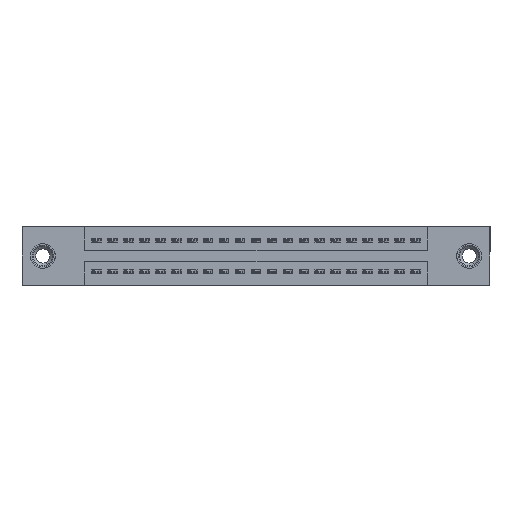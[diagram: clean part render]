
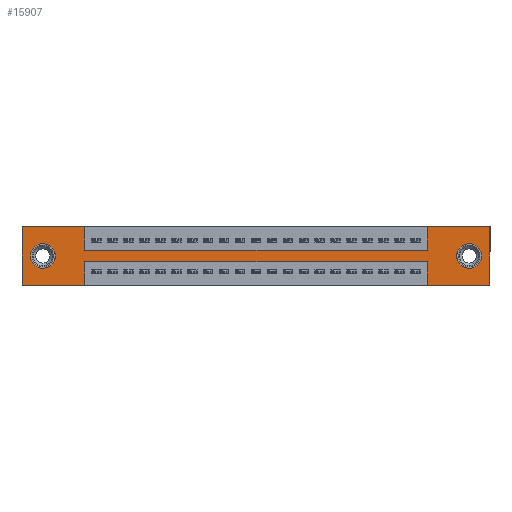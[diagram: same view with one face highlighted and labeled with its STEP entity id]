
A CAD part, front view. The second image highlights one B-rep face of the part: STEP entity #15907.
In plain terms, the highlighted planar face has unit normal (0, -1, 0).
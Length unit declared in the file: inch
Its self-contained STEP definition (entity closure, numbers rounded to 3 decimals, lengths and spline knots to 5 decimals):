
#292 = DIRECTION ( 'NONE',  ( 0., 0., -1. ) ) ;
#305 = CARTESIAN_POINT ( 'NONE',  ( 0., 0., -0.37 ) ) ;
#357 = CARTESIAN_POINT ( 'NONE',  ( 0., 0., 0. ) ) ;
#392 = CARTESIAN_POINT ( 'NONE',  ( 2.5425, 0., 0. ) ) ;
#472 = DIRECTION ( 'NONE',  ( 0., 0., -1. ) ) ;
#495 = CARTESIAN_POINT ( 'NONE',  ( 2.935, 0., 0. ) ) ;
#607 = DIRECTION ( 'NONE',  ( 1., 0., 0. ) ) ;
#788 = EDGE_CURVE ( 'NONE', #6210, #15255, #9337, .T. ) ;
#856 = CARTESIAN_POINT ( 'NONE',  ( 0.13, 0., -0.263 ) ) ;
#1022 = AXIS2_PLACEMENT_3D ( 'NONE', #18558, #13735, #15409 ) ;
#1032 = CIRCLE ( 'NONE', #16692, 0.078 ) ;
#1078 = VECTOR ( 'NONE', #10219, 39.37008 ) ;
#1104 = ORIENTED_EDGE ( 'NONE', *, *, #15872, .F. ) ;
#1366 = EDGE_CURVE ( 'NONE', #14508, #17656, #20268, .T. ) ;
#1466 = DIRECTION ( 'NONE',  ( 0., 0., 1. ) ) ;
#1497 = EDGE_CURVE ( 'NONE', #8282, #8139, #3645, .T. ) ;
#1965 = CARTESIAN_POINT ( 'NONE',  ( 0.3925, 0., -0.22 ) ) ;
#2150 = EDGE_CURVE ( 'NONE', #5523, #16238, #2598, .T. ) ;
#2354 = VERTEX_POINT ( 'NONE', #9370 ) ;
#2570 = ORIENTED_EDGE ( 'NONE', *, *, #788, .F. ) ;
#2598 = LINE ( 'NONE', #8615, #6475 ) ;
#2851 = EDGE_CURVE ( 'NONE', #16183, #10274, #19952, .T. ) ;
#3087 = CARTESIAN_POINT ( 'NONE',  ( 0.13, 0., -0.185 ) ) ;
#3565 = DIRECTION ( 'NONE',  ( 0., 0., -1. ) ) ;
#3645 = LINE ( 'NONE', #14074, #12171 ) ;
#3792 = VECTOR ( 'NONE', #1466, 39.37008 ) ;
#3975 = ORIENTED_EDGE ( 'NONE', *, *, #12436, .F. ) ;
#4322 = ORIENTED_EDGE ( 'NONE', *, *, #5326, .T. ) ;
#4615 = CARTESIAN_POINT ( 'NONE',  ( 0.3925, 0., -0.37 ) ) ;
#4636 = EDGE_CURVE ( 'NONE', #20492, #5523, #18578, .T. ) ;
#4645 = EDGE_LOOP ( 'NONE', ( #10405, #4322 ) ) ;
#4746 = VERTEX_POINT ( 'NONE', #856 ) ;
#4771 = CARTESIAN_POINT ( 'NONE',  ( 2.5425, 0., -0.37 ) ) ;
#4886 = CIRCLE ( 'NONE', #1022, 0.078 ) ;
#5216 = CARTESIAN_POINT ( 'NONE',  ( 2.5425, 0., -0.22 ) ) ;
#5326 = EDGE_CURVE ( 'NONE', #17656, #14508, #20364, .T. ) ;
#5474 = AXIS2_PLACEMENT_3D ( 'NONE', #8737, #10388, #292 ) ;
#5523 = VERTEX_POINT ( 'NONE', #4615 ) ;
#5547 = CARTESIAN_POINT ( 'NONE',  ( 2.5425, 0., 0. ) ) ;
#5802 = LINE ( 'NONE', #18113, #21106 ) ;
#6210 = VERTEX_POINT ( 'NONE', #5547 ) ;
#6363 = VERTEX_POINT ( 'NONE', #357 ) ;
#6380 = VECTOR ( 'NONE', #10973, 39.37008 ) ;
#6475 = VECTOR ( 'NONE', #10263, 39.37008 ) ;
#6629 = VECTOR ( 'NONE', #15482, 39.37008 ) ;
#6963 = VECTOR ( 'NONE', #11293, 39.37008 ) ;
#6988 = EDGE_LOOP ( 'NONE', ( #13357, #9820 ) ) ;
#7296 = ORIENTED_EDGE ( 'NONE', *, *, #12013, .F. ) ;
#7413 = LINE ( 'NONE', #19263, #6380 ) ;
#8139 = VERTEX_POINT ( 'NONE', #5216 ) ;
#8282 = VERTEX_POINT ( 'NONE', #4771 ) ;
#8615 = CARTESIAN_POINT ( 'NONE',  ( 0., 0., -0.37 ) ) ;
#8737 = CARTESIAN_POINT ( 'NONE',  ( 2.805, 0., -0.185 ) ) ;
#9034 = CARTESIAN_POINT ( 'NONE',  ( 0.3925, 0., 0. ) ) ;
#9337 = LINE ( 'NONE', #20199, #1078 ) ;
#9370 = CARTESIAN_POINT ( 'NONE',  ( 0.13, 0., -0.107 ) ) ;
#9375 = EDGE_CURVE ( 'NONE', #8139, #20492, #17091, .T. ) ;
#9593 = ORIENTED_EDGE ( 'NONE', *, *, #4636, .F. ) ;
#9820 = ORIENTED_EDGE ( 'NONE', *, *, #17689, .T. ) ;
#9832 = CARTESIAN_POINT ( 'NONE',  ( 0.3925, 0., -0.22 ) ) ;
#10169 = FACE_OUTER_BOUND ( 'NONE', #18717, .T. ) ;
#10219 = DIRECTION ( 'NONE',  ( 1., 0., 0. ) ) ;
#10263 = DIRECTION ( 'NONE',  ( -1., 0., 0. ) ) ;
#10274 = VERTEX_POINT ( 'NONE', #19310 ) ;
#10388 = DIRECTION ( 'NONE',  ( 0., 1., 0. ) ) ;
#10405 = ORIENTED_EDGE ( 'NONE', *, *, #1366, .T. ) ;
#10420 = VECTOR ( 'NONE', #3565, 39.37008 ) ;
#10530 = PLANE ( 'NONE',  #21391 ) ;
#10772 = ORIENTED_EDGE ( 'NONE', *, *, #2150, .F. ) ;
#10973 = DIRECTION ( 'NONE',  ( 0., 0., -1. ) ) ;
#10995 = CARTESIAN_POINT ( 'NONE',  ( 0.3925, 0., -0.15 ) ) ;
#11293 = DIRECTION ( 'NONE',  ( -1., 0., 0. ) ) ;
#12013 = EDGE_CURVE ( 'NONE', #16238, #6363, #12051, .T. ) ;
#12051 = LINE ( 'NONE', #13204, #3792 ) ;
#12171 = VECTOR ( 'NONE', #17147, 39.37008 ) ;
#12197 = EDGE_CURVE ( 'NONE', #18510, #16183, #7413, .T. ) ;
#12329 = LINE ( 'NONE', #17244, #20170 ) ;
#12436 = EDGE_CURVE ( 'NONE', #10274, #6210, #15404, .T. ) ;
#13119 = DIRECTION ( 'NONE',  ( 0., 1., 0. ) ) ;
#13204 = CARTESIAN_POINT ( 'NONE',  ( 0., 0., 0. ) ) ;
#13357 = ORIENTED_EDGE ( 'NONE', *, *, #18985, .T. ) ;
#13735 = DIRECTION ( 'NONE',  ( 0., 1., 0. ) ) ;
#14074 = CARTESIAN_POINT ( 'NONE',  ( 2.5425, 0., -0.37 ) ) ;
#14119 = VERTEX_POINT ( 'NONE', #19555 ) ;
#14134 = VECTOR ( 'NONE', #472, 39.37008 ) ;
#14342 = ORIENTED_EDGE ( 'NONE', *, *, #2851, .F. ) ;
#14503 = DIRECTION ( 'NONE',  ( 0., 0., 1. ) ) ;
#14508 = VERTEX_POINT ( 'NONE', #18711 ) ;
#14609 = CARTESIAN_POINT ( 'NONE',  ( 2.805, 0., -0.185 ) ) ;
#14839 = LINE ( 'NONE', #18282, #10420 ) ;
#15024 = CARTESIAN_POINT ( 'NONE',  ( 0., 0., -0.37 ) ) ;
#15219 = VECTOR ( 'NONE', #19822, 39.37008 ) ;
#15255 = VERTEX_POINT ( 'NONE', #495 ) ;
#15404 = LINE ( 'NONE', #392, #6629 ) ;
#15409 = DIRECTION ( 'NONE',  ( 0., 0., 1. ) ) ;
#15412 = CARTESIAN_POINT ( 'NONE',  ( 0.3925, 0., -0.37 ) ) ;
#15482 = DIRECTION ( 'NONE',  ( 0., 0., 1. ) ) ;
#15551 = EDGE_CURVE ( 'NONE', #15255, #14119, #14839, .T. ) ;
#15631 = FACE_BOUND ( 'NONE', #4645, .T. ) ;
#15738 = ORIENTED_EDGE ( 'NONE', *, *, #15551, .F. ) ;
#15872 = EDGE_CURVE ( 'NONE', #6363, #18510, #5802, .T. ) ;
#15907 = ADVANCED_FACE ( 'NONE', ( #15631, #19842, #10169 ), #10530, .T. ) ;
#16183 = VERTEX_POINT ( 'NONE', #10995 ) ;
#16238 = VERTEX_POINT ( 'NONE', #305 ) ;
#16351 = AXIS2_PLACEMENT_3D ( 'NONE', #14609, #16709, #21498 ) ;
#16692 = AXIS2_PLACEMENT_3D ( 'NONE', #3087, #13119, #14503 ) ;
#16709 = DIRECTION ( 'NONE',  ( 0., 1., 0. ) ) ;
#17091 = LINE ( 'NONE', #9832, #6963 ) ;
#17147 = DIRECTION ( 'NONE',  ( 0., 0., 1. ) ) ;
#17244 = CARTESIAN_POINT ( 'NONE',  ( 0., 0., -0.37 ) ) ;
#17310 = DIRECTION ( 'NONE',  ( -1., 0., 0. ) ) ;
#17656 = VERTEX_POINT ( 'NONE', #20778 ) ;
#17689 = EDGE_CURVE ( 'NONE', #4746, #2354, #1032, .T. ) ;
#17830 = CARTESIAN_POINT ( 'NONE',  ( 0.3925, 0., -0.15 ) ) ;
#18113 = CARTESIAN_POINT ( 'NONE',  ( 0., 0., 0. ) ) ;
#18282 = CARTESIAN_POINT ( 'NONE',  ( 2.935, 0., 0. ) ) ;
#18334 = ORIENTED_EDGE ( 'NONE', *, *, #1497, .F. ) ;
#18510 = VERTEX_POINT ( 'NONE', #9034 ) ;
#18558 = CARTESIAN_POINT ( 'NONE',  ( 0.13, 0., -0.185 ) ) ;
#18578 = LINE ( 'NONE', #15412, #14134 ) ;
#18711 = CARTESIAN_POINT ( 'NONE',  ( 2.805, 0., -0.107 ) ) ;
#18717 = EDGE_LOOP ( 'NONE', ( #9593, #21372, #18334, #19987, #15738, #2570, #3975, #14342, #19672, #1104, #7296, #10772 ) ) ;
#18985 = EDGE_CURVE ( 'NONE', #2354, #4746, #4886, .T. ) ;
#19263 = CARTESIAN_POINT ( 'NONE',  ( 0.3925, 0., 0. ) ) ;
#19310 = CARTESIAN_POINT ( 'NONE',  ( 2.5425, 0., -0.15 ) ) ;
#19555 = CARTESIAN_POINT ( 'NONE',  ( 2.935, 0., -0.37 ) ) ;
#19672 = ORIENTED_EDGE ( 'NONE', *, *, #12197, .F. ) ;
#19749 = DIRECTION ( 'NONE',  ( 0., -1., 0. ) ) ;
#19822 = DIRECTION ( 'NONE',  ( 1., 0., 0. ) ) ;
#19842 = FACE_BOUND ( 'NONE', #6988, .T. ) ;
#19952 = LINE ( 'NONE', #17830, #15219 ) ;
#19987 = ORIENTED_EDGE ( 'NONE', *, *, #20449, .F. ) ;
#20170 = VECTOR ( 'NONE', #17310, 39.37008 ) ;
#20199 = CARTESIAN_POINT ( 'NONE',  ( 0., 0., 0. ) ) ;
#20268 = CIRCLE ( 'NONE', #5474, 0.078 ) ;
#20364 = CIRCLE ( 'NONE', #16351, 0.078 ) ;
#20449 = EDGE_CURVE ( 'NONE', #14119, #8282, #12329, .T. ) ;
#20492 = VERTEX_POINT ( 'NONE', #1965 ) ;
#20778 = CARTESIAN_POINT ( 'NONE',  ( 2.805, 0., -0.263 ) ) ;
#21106 = VECTOR ( 'NONE', #607, 39.37008 ) ;
#21245 = DIRECTION ( 'NONE',  ( 0., 0., -1. ) ) ;
#21372 = ORIENTED_EDGE ( 'NONE', *, *, #9375, .F. ) ;
#21391 = AXIS2_PLACEMENT_3D ( 'NONE', #15024, #19749, #21245 ) ;
#21498 = DIRECTION ( 'NONE',  ( 0., 0., -1. ) ) ;
